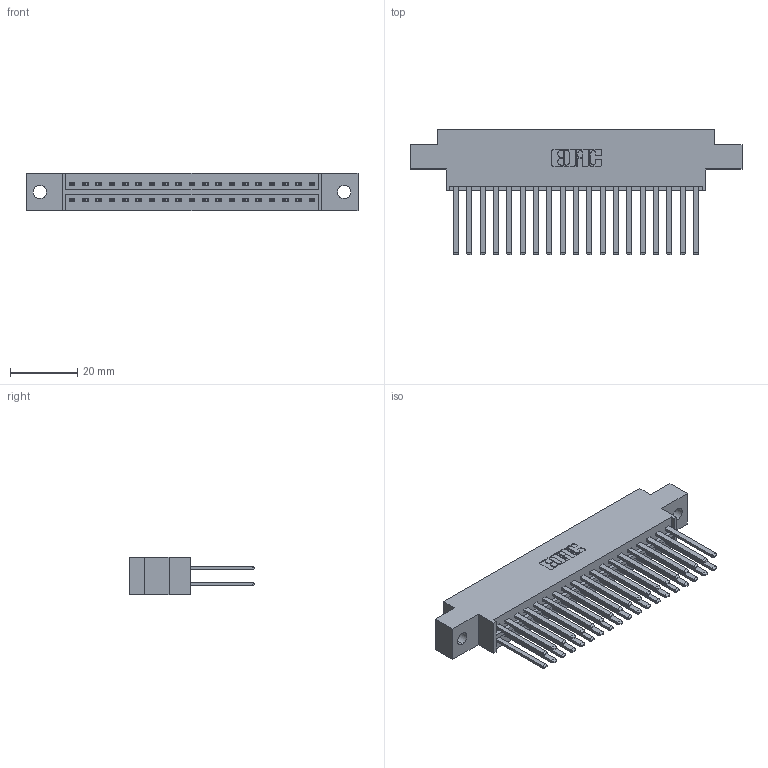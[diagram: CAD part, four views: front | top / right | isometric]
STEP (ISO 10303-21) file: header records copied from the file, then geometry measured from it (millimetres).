
FILE_DESCRIPTION (( 'STEP AP203' ), '1' );
FILE_NAME ('336-038-541-804.STEP', '2020-08-07T23:05:05', ( '' ), ( '' ), 'SwSTEP 2.0', 'SolidWorks 2020', '' );
FILE_SCHEMA (( 'CONFIG_CONTROL_DESIGN' ));
Length unit declared in the file: inch
Products named in the file (3): 336-290-001_336-290-541; 336-038-541-804; 336 Part_Offset - .156 Dia - TH
Assembly tree (39 placements, depth 2):
  336-038-541-804
    336 Part_Offset - .156 Dia - TH
    336-290-001_336-290-541  x38
Bounding box: 98.68 x 37.34 x 11.1 mm (x, y, z)
Volume: 14395 mm3; surface area: 17818.7 mm2
Topology: 39 solids, 39 shells, 1714 faces, 5149 edges, 3406 vertices
Faces by surface type: plane 1062, cylinder 652
Entity records: 17560 total; most frequent: CARTESIAN_POINT 3061, ORIENTED_EDGE 2898, DIRECTION 2549, EDGE_CURVE 1449, VECTOR 1317, LINE 1317, VERTEX_POINT 964, AXIS2_PLACEMENT_3D 616
